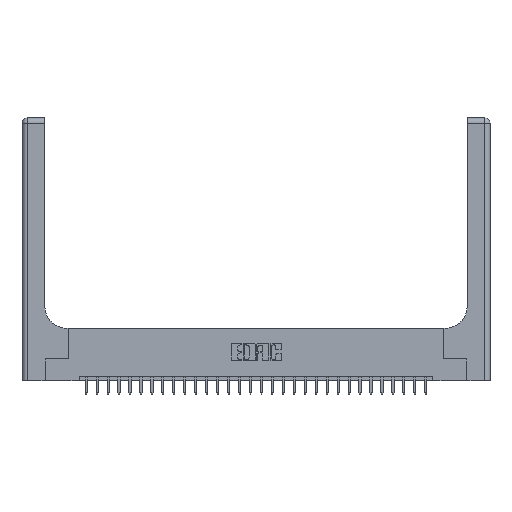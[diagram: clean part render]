
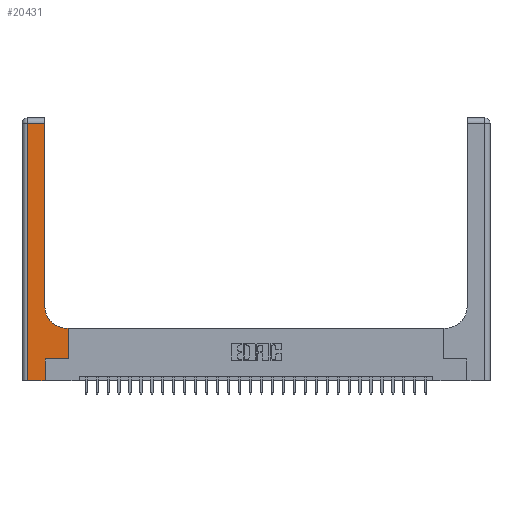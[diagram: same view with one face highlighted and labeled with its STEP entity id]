
A CAD part, top view. The second image highlights one B-rep face of the part: STEP entity #20431.
In plain terms, the highlighted planar face has unit normal (0, 0, 1).
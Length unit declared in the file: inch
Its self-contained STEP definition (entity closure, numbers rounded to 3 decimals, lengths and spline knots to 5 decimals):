
#53 = CARTESIAN_POINT ( 'NONE',  ( 0., 0., 0.37 ) ) ;
#407 = DIRECTION ( 'NONE',  ( -1., 0., 0. ) ) ;
#1275 = PLANE ( 'NONE',  #9506 ) ;
#1798 = CARTESIAN_POINT ( 'NONE',  ( 0.265, 0.25, 0.37 ) ) ;
#2054 = LINE ( 'NONE', #53, #10765 ) ;
#2116 = EDGE_CURVE ( 'NONE', #8582, #15635, #2054, .T. ) ;
#2226 = DIRECTION ( 'NONE',  ( 0., 1., 0. ) ) ;
#2589 = DIRECTION ( 'NONE',  ( 0., -1., 0. ) ) ;
#3078 = ORIENTED_EDGE ( 'NONE', *, *, #13150, .T. ) ;
#3185 = EDGE_CURVE ( 'NONE', #22507, #5315, #24385, .T. ) ;
#3200 = LINE ( 'NONE', #20379, #24879 ) ;
#3928 = ORIENTED_EDGE ( 'NONE', *, *, #24777, .T. ) ;
#4212 = LINE ( 'NONE', #10430, #22169 ) ;
#4704 = LINE ( 'NONE', #21882, #20465 ) ;
#5195 = CARTESIAN_POINT ( 'NONE',  ( 0.26, 2.94, 0.37 ) ) ;
#5315 = VERTEX_POINT ( 'NONE', #9843 ) ;
#5744 = DIRECTION ( 'NONE',  ( 0., 1., 0. ) ) ;
#6242 = VERTEX_POINT ( 'NONE', #25917 ) ;
#6328 = ORIENTED_EDGE ( 'NONE', *, *, #24294, .T. ) ;
#6407 = EDGE_LOOP ( 'NONE', ( #6328, #9293, #7936, #11696, #17893, #17858, #3928, #26541, #3078 ) ) ;
#6935 = DIRECTION ( 'NONE',  ( 1., 0., 0. ) ) ;
#7293 = DIRECTION ( 'NONE',  ( 0., 1., 0. ) ) ;
#7489 = VERTEX_POINT ( 'NONE', #12832 ) ;
#7490 = AXIS2_PLACEMENT_3D ( 'NONE', #15103, #10763, #6935 ) ;
#7936 = ORIENTED_EDGE ( 'NONE', *, *, #26697, .T. ) ;
#8144 = CARTESIAN_POINT ( 'NONE',  ( 0.528, 0.25, 0.37 ) ) ;
#8299 = DIRECTION ( 'NONE',  ( 1., 0., 0. ) ) ;
#8561 = CARTESIAN_POINT ( 'NONE',  ( 0.06, 0., 0.37 ) ) ;
#8582 = VERTEX_POINT ( 'NONE', #8561 ) ;
#8689 = CARTESIAN_POINT ( 'NONE',  ( 0.265, 0., 0.37 ) ) ;
#9293 = ORIENTED_EDGE ( 'NONE', *, *, #3185, .T. ) ;
#9491 = CARTESIAN_POINT ( 'NONE',  ( 0., 2.94, 0.37 ) ) ;
#9506 = AXIS2_PLACEMENT_3D ( 'NONE', #22570, #27350, #16250 ) ;
#9554 = EDGE_CURVE ( 'NONE', #15635, #6242, #4212, .T. ) ;
#9843 = CARTESIAN_POINT ( 'NONE',  ( 0.06, 2.94, 0.37 ) ) ;
#9885 = CARTESIAN_POINT ( 'NONE',  ( 0.26, 0.85, 0.37 ) ) ;
#10430 = CARTESIAN_POINT ( 'NONE',  ( 0.265, 0., 0.37 ) ) ;
#10763 = DIRECTION ( 'NONE',  ( 0., 0., -1. ) ) ;
#10765 = VECTOR ( 'NONE', #27866, 39.37008 ) ;
#11412 = VECTOR ( 'NONE', #5744, 39.37008 ) ;
#11696 = ORIENTED_EDGE ( 'NONE', *, *, #2116, .T. ) ;
#11890 = FACE_OUTER_BOUND ( 'NONE', #6407, .T. ) ;
#12832 = CARTESIAN_POINT ( 'NONE',  ( 0.528, 0.25, 0.37 ) ) ;
#13150 = EDGE_CURVE ( 'NONE', #18511, #14938, #23678, .T. ) ;
#13386 = CARTESIAN_POINT ( 'NONE',  ( 0.51, 0.6, 0.37 ) ) ;
#14628 = LINE ( 'NONE', #1798, #26810 ) ;
#14935 = EDGE_CURVE ( 'NONE', #6242, #7489, #14628, .T. ) ;
#14938 = VERTEX_POINT ( 'NONE', #9885 ) ;
#15103 = CARTESIAN_POINT ( 'NONE',  ( 0.51, 0.85, 0.37 ) ) ;
#15635 = VERTEX_POINT ( 'NONE', #8689 ) ;
#16250 = DIRECTION ( 'NONE',  ( -1., 0., 0. ) ) ;
#16443 = LINE ( 'NONE', #8144, #11412 ) ;
#17483 = VECTOR ( 'NONE', #407, 39.37008 ) ;
#17541 = VERTEX_POINT ( 'NONE', #27293 ) ;
#17720 = DIRECTION ( 'NONE',  ( -1., 0., 0. ) ) ;
#17858 = ORIENTED_EDGE ( 'NONE', *, *, #14935, .T. ) ;
#17893 = ORIENTED_EDGE ( 'NONE', *, *, #9554, .T. ) ;
#18511 = VERTEX_POINT ( 'NONE', #13386 ) ;
#19998 = CARTESIAN_POINT ( 'NONE',  ( 0.26, 0.6, 0.37 ) ) ;
#20379 = CARTESIAN_POINT ( 'NONE',  ( 0.26, 3., 0.37 ) ) ;
#20431 = ADVANCED_FACE ( 'NONE', ( #11890 ), #1275, .F. ) ;
#20465 = VECTOR ( 'NONE', #2589, 39.37008 ) ;
#21882 = CARTESIAN_POINT ( 'NONE',  ( 0.06, 3., 0.37 ) ) ;
#22169 = VECTOR ( 'NONE', #2226, 39.37008 ) ;
#22371 = EDGE_CURVE ( 'NONE', #17541, #18511, #26043, .T. ) ;
#22507 = VERTEX_POINT ( 'NONE', #5195 ) ;
#22570 = CARTESIAN_POINT ( 'NONE',  ( 0., 3., 0.37 ) ) ;
#23678 = CIRCLE ( 'NONE', #7490, 0.25 ) ;
#24294 = EDGE_CURVE ( 'NONE', #14938, #22507, #3200, .T. ) ;
#24385 = LINE ( 'NONE', #9491, #17483 ) ;
#24777 = EDGE_CURVE ( 'NONE', #7489, #17541, #16443, .T. ) ;
#24879 = VECTOR ( 'NONE', #7293, 39.37008 ) ;
#25917 = CARTESIAN_POINT ( 'NONE',  ( 0.265, 0.25, 0.37 ) ) ;
#26043 = LINE ( 'NONE', #19998, #27463 ) ;
#26541 = ORIENTED_EDGE ( 'NONE', *, *, #22371, .T. ) ;
#26697 = EDGE_CURVE ( 'NONE', #5315, #8582, #4704, .T. ) ;
#26810 = VECTOR ( 'NONE', #8299, 39.37008 ) ;
#27293 = CARTESIAN_POINT ( 'NONE',  ( 0.528, 0.6, 0.37 ) ) ;
#27350 = DIRECTION ( 'NONE',  ( 0., 0., -1. ) ) ;
#27463 = VECTOR ( 'NONE', #17720, 39.37008 ) ;
#27866 = DIRECTION ( 'NONE',  ( 1., 0., 0. ) ) ;
